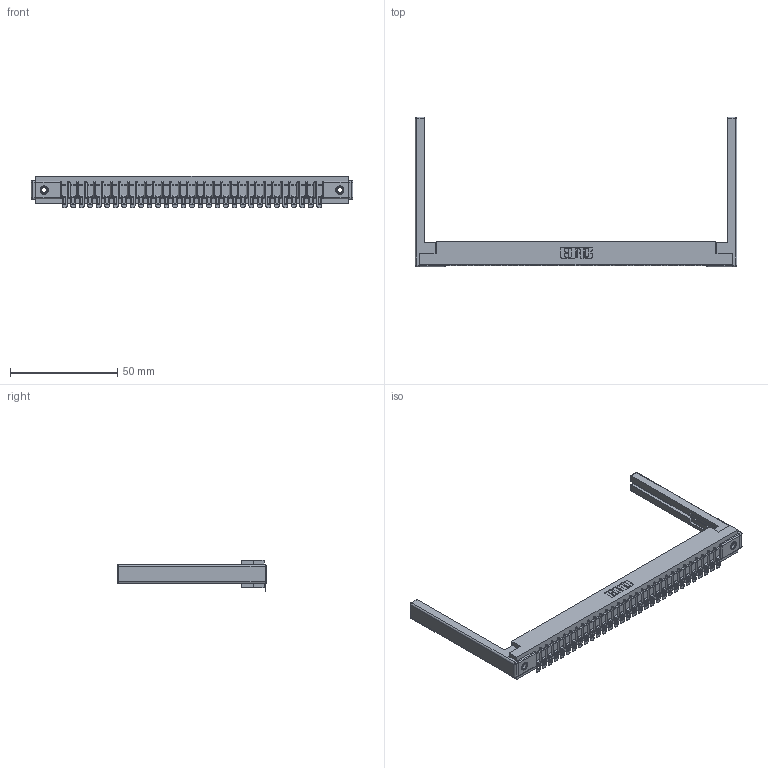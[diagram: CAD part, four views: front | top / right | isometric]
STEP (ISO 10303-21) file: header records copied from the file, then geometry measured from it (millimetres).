
FILE_DESCRIPTION (( 'STEP AP203' ), '1' );
FILE_NAME ('307-031-554-168.STEP', '2019-09-05T05:01:01', ( '' ), ( '' ), 'SwSTEP 2.0', 'SolidWorks 2016', '' );
FILE_SCHEMA (( 'CONFIG_CONTROL_DESIGN' ));
Length unit declared in the file: inch
Products named in the file (5): 307-290-002_554; 307-220-068; 307-031-554-168; 307 Part_.156 Dia Mounting Holes; 345-250-001_345-250-001-102
Assembly tree (36 placements, depth 2):
  307-031-554-168
    307 Part_.156 Dia Mounting Holes
    307-290-002_554  x31
    307-220-068  x2
    345-250-001_345-250-001-102  x2
Bounding box: 150.27 x 69.98 x 14.52 mm (x, y, z)
Volume: 20387.2 mm3; surface area: 23969.5 mm2
Topology: 36 solids, 36 shells, 2815 faces, 8556 edges, 5596 vertices
Faces by surface type: plane 1584, cylinder 1143, sphere 72, cone 12, torus 4
Entity records: 31656 total; most frequent: CARTESIAN_POINT 5303, ORIENTED_EDGE 5282, DIRECTION 5181, EDGE_CURVE 2641, VECTOR 2009, LINE 2009, VERTEX_POINT 1708, AXIS2_PLACEMENT_3D 1586
